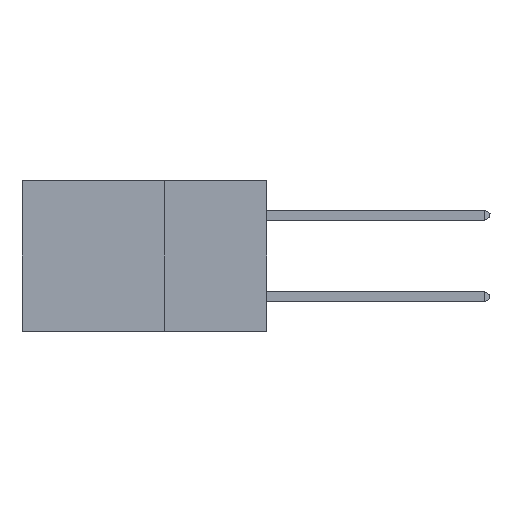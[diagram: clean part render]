
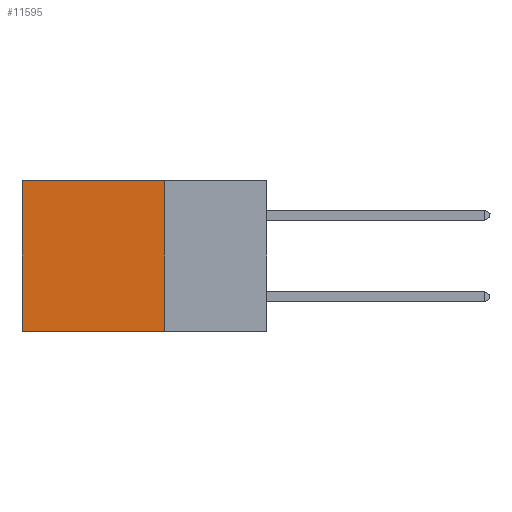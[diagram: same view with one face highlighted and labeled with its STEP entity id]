
A CAD part, left-side view. The second image highlights one B-rep face of the part: STEP entity #11595.
In plain terms, the highlighted planar face has unit normal (-1, 0, 0).
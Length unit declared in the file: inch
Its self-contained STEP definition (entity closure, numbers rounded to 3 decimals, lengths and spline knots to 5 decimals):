
#431 = DIRECTION ( 'NONE',  ( 0., 0., -1. ) ) ;
#1053 = VERTEX_POINT ( 'NONE', #7357 ) ;
#1354 = VECTOR ( 'NONE', #10082, 39.37008 ) ;
#1675 = CARTESIAN_POINT ( 'NONE',  ( 0.2875, 0.25, 0. ) ) ;
#2180 = PLANE ( 'NONE',  #12399 ) ;
#2706 = CARTESIAN_POINT ( 'NONE',  ( 0.2875, 0.25, -0.37 ) ) ;
#3217 = EDGE_CURVE ( 'NONE', #7552, #6647, #11547, .T. ) ;
#3930 = DIRECTION ( 'NONE',  ( 0., 1., 0. ) ) ;
#4005 = EDGE_CURVE ( 'NONE', #6647, #1053, #10299, .T. ) ;
#4249 = ORIENTED_EDGE ( 'NONE', *, *, #4005, .T. ) ;
#4577 = DIRECTION ( 'NONE',  ( 1., 0., 0. ) ) ;
#5064 = CARTESIAN_POINT ( 'NONE',  ( 0.2875, 0.25, 0. ) ) ;
#5261 = ORIENTED_EDGE ( 'NONE', *, *, #11840, .F. ) ;
#5594 = EDGE_LOOP ( 'NONE', ( #4249, #5261, #7151, #7877 ) ) ;
#6114 = CARTESIAN_POINT ( 'NONE',  ( 0.2875, 0.6, 0. ) ) ;
#6647 = VERTEX_POINT ( 'NONE', #6114 ) ;
#7151 = ORIENTED_EDGE ( 'NONE', *, *, #12601, .F. ) ;
#7301 = VECTOR ( 'NONE', #3930, 39.37008 ) ;
#7357 = CARTESIAN_POINT ( 'NONE',  ( 0.2875, 0.6, -0.37 ) ) ;
#7552 = VERTEX_POINT ( 'NONE', #5064 ) ;
#7877 = ORIENTED_EDGE ( 'NONE', *, *, #3217, .T. ) ;
#8192 = DIRECTION ( 'NONE',  ( 0., 1., 0. ) ) ;
#8195 = FACE_OUTER_BOUND ( 'NONE', #5594, .T. ) ;
#8673 = CARTESIAN_POINT ( 'NONE',  ( 0.2875, 0.25, 0. ) ) ;
#9761 = LINE ( 'NONE', #1675, #12052 ) ;
#9935 = CARTESIAN_POINT ( 'NONE',  ( 0.2875, 0.6, 0. ) ) ;
#10082 = DIRECTION ( 'NONE',  ( 0., 0., -1. ) ) ;
#10281 = CARTESIAN_POINT ( 'NONE',  ( 0.2875, 0.25, -0.37 ) ) ;
#10299 = LINE ( 'NONE', #9935, #1354 ) ;
#11396 = CARTESIAN_POINT ( 'NONE',  ( 0.2875, 0.25, 0. ) ) ;
#11547 = LINE ( 'NONE', #8673, #14053 ) ;
#11595 = ADVANCED_FACE ( 'NONE', ( #8195 ), #2180, .F. ) ;
#11840 = EDGE_CURVE ( 'NONE', #14499, #1053, #13248, .T. ) ;
#12052 = VECTOR ( 'NONE', #431, 39.37008 ) ;
#12399 = AXIS2_PLACEMENT_3D ( 'NONE', #11396, #4577, #12579 ) ;
#12579 = DIRECTION ( 'NONE',  ( 0., 0., -1. ) ) ;
#12601 = EDGE_CURVE ( 'NONE', #7552, #14499, #9761, .T. ) ;
#13248 = LINE ( 'NONE', #2706, #7301 ) ;
#14053 = VECTOR ( 'NONE', #8192, 39.37008 ) ;
#14499 = VERTEX_POINT ( 'NONE', #10281 ) ;
